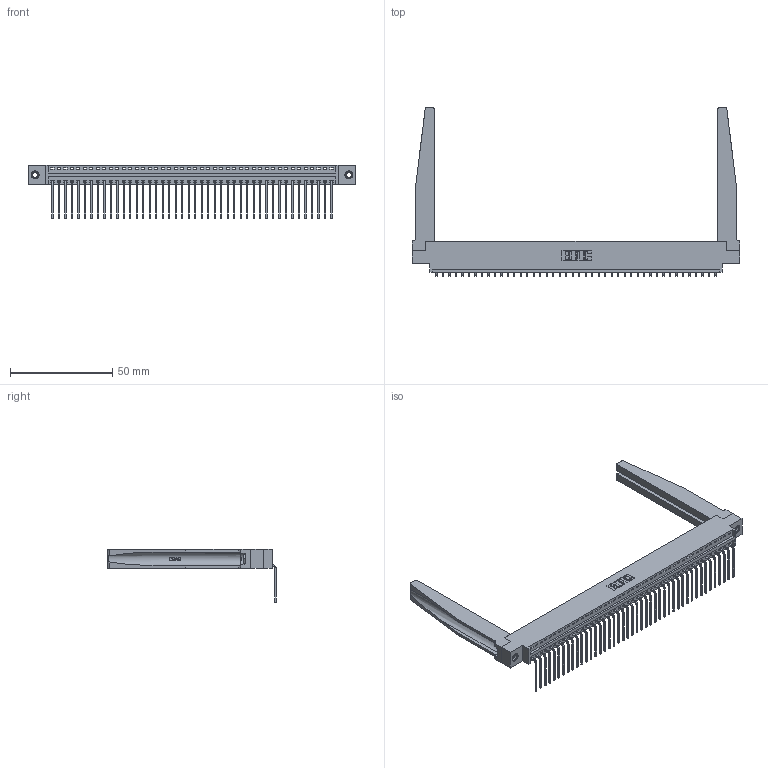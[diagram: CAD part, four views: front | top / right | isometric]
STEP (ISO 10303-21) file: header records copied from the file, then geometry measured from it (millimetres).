
FILE_DESCRIPTION (( 'STEP AP203' ), '1' );
FILE_NAME ('396-044-559-678.STEP', '2019-10-31T23:12:19', ( '' ), ( '' ), 'SwSTEP 2.0', 'SolidWorks 2016', '' );
FILE_SCHEMA (( 'CONFIG_CONTROL_DESIGN' ));
Length unit declared in the file: inch
Products named in the file (5): 346 Part_0.170 Offset - 0.156 Dia-TH; 345-292-001_558 559 Tail - 1; 346-220-078_345-220-078; 345-250-001_345-250-001-102; 396-044-559-678
Assembly tree (49 placements, depth 2):
  396-044-559-678
    346 Part_0.170 Offset - 0.156 Dia-TH
    345-292-001_558 559 Tail - 1  x44
    346-220-078_345-220-078  x2
    345-250-001_345-250-001-102  x2
Bounding box: 160.27 x 82.36 x 26.16 mm (x, y, z)
Volume: 22256.4 mm3; surface area: 26779 mm2
Topology: 49 solids, 49 shells, 3000 faces, 8957 edges, 5902 vertices
Faces by surface type: plane 2070, cylinder 878, bspline 36, cone 12, torus 4
Entity records: 32002 total; most frequent: CARTESIAN_POINT 6399, ORIENTED_EDGE 5266, DIRECTION 4627, EDGE_CURVE 2633, LINE 2231, VECTOR 2231, VERTEX_POINT 1748, AXIS2_PLACEMENT_3D 1198
